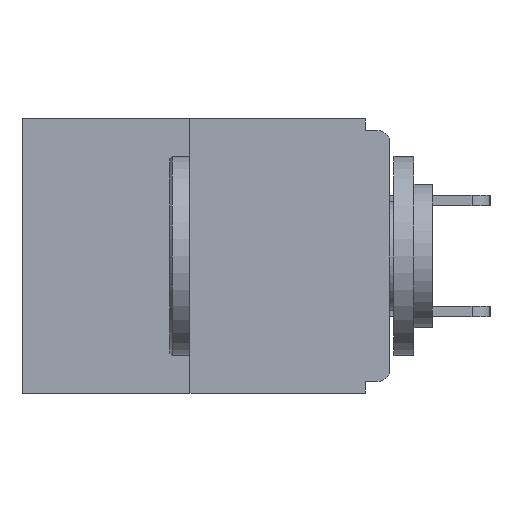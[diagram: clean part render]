
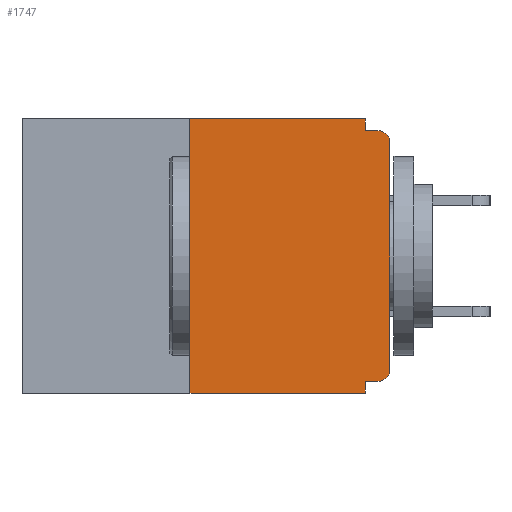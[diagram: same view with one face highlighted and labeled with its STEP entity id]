
A CAD part, left-side view. The second image highlights one B-rep face of the part: STEP entity #1747.
In plain terms, the highlighted planar face has unit normal (-1, 0, 0).
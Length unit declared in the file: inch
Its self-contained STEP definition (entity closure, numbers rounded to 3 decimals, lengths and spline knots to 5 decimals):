
#336 = CARTESIAN_POINT ( 'NONE',  ( 0., 0., 0. ) ) ;
#378 = EDGE_CURVE ( 'NONE', #7450, #7060, #9176, .T. ) ;
#493 = ORIENTED_EDGE ( 'NONE', *, *, #6042, .T. ) ;
#903 = CARTESIAN_POINT ( 'NONE',  ( 0., 0.015, -0.328 ) ) ;
#1571 = AXIS2_PLACEMENT_3D ( 'NONE', #9705, #12685, #5199 ) ;
#1747 = ADVANCED_FACE ( 'NONE', ( #12471 ), #16824, .F. ) ;
#1782 = ORIENTED_EDGE ( 'NONE', *, *, #12247, .F. ) ;
#1914 = VECTOR ( 'NONE', #4579, 39.37008 ) ;
#2179 = ORIENTED_EDGE ( 'NONE', *, *, #2939, .T. ) ;
#2742 = CARTESIAN_POINT ( 'NONE',  ( 0., 0.031, 0. ) ) ;
#2891 = VECTOR ( 'NONE', #10125, 39.37008 ) ;
#2907 = ORIENTED_EDGE ( 'NONE', *, *, #17609, .F. ) ;
#2908 = CIRCLE ( 'NONE', #16454, 0.015 ) ;
#2939 = EDGE_CURVE ( 'NONE', #8677, #5398, #2908, .T. ) ;
#3215 = DIRECTION ( 'NONE',  ( 0., -1., 0. ) ) ;
#3531 = LINE ( 'NONE', #6331, #19119 ) ;
#3634 = EDGE_LOOP ( 'NONE', ( #19291, #2907, #9939, #10907, #9017, #2179, #13256, #493, #1782, #12936 ) ) ;
#3779 = LINE ( 'NONE', #4654, #7376 ) ;
#3842 = VERTEX_POINT ( 'NONE', #15875 ) ;
#4537 = VERTEX_POINT ( 'NONE', #10192 ) ;
#4558 = VERTEX_POINT ( 'NONE', #11864 ) ;
#4579 = DIRECTION ( 'NONE',  ( 0., 1., 0. ) ) ;
#4654 = CARTESIAN_POINT ( 'NONE',  ( 0., 0.46, -0.343 ) ) ;
#5199 = DIRECTION ( 'NONE',  ( 0., 0., -1. ) ) ;
#5398 = VERTEX_POINT ( 'NONE', #12052 ) ;
#5694 = VERTEX_POINT ( 'NONE', #8526 ) ;
#5939 = LINE ( 'NONE', #18238, #1914 ) ;
#6042 = EDGE_CURVE ( 'NONE', #4558, #12372, #14712, .T. ) ;
#6188 = DIRECTION ( 'NONE',  ( 0., -1., 0. ) ) ;
#6326 = DIRECTION ( 'NONE',  ( -1., 0., 0. ) ) ;
#6331 = CARTESIAN_POINT ( 'NONE',  ( 0., 0., -0.015 ) ) ;
#6451 = LINE ( 'NONE', #18977, #2891 ) ;
#6812 = EDGE_CURVE ( 'NONE', #5398, #4558, #17959, .T. ) ;
#7060 = VERTEX_POINT ( 'NONE', #12876 ) ;
#7376 = VECTOR ( 'NONE', #6188, 39.37008 ) ;
#7450 = VERTEX_POINT ( 'NONE', #12485 ) ;
#7840 = VECTOR ( 'NONE', #17585, 39.37008 ) ;
#7907 = DIRECTION ( 'NONE',  ( 0., 0., -1. ) ) ;
#8076 = LINE ( 'NONE', #8389, #7840 ) ;
#8389 = CARTESIAN_POINT ( 'NONE',  ( 0., 0.25, 0. ) ) ;
#8526 = CARTESIAN_POINT ( 'NONE',  ( 0., 0.25, -0.343 ) ) ;
#8677 = VERTEX_POINT ( 'NONE', #903 ) ;
#8842 = LINE ( 'NONE', #2742, #9540 ) ;
#9017 = ORIENTED_EDGE ( 'NONE', *, *, #17894, .F. ) ;
#9176 = LINE ( 'NONE', #15212, #18813 ) ;
#9540 = VECTOR ( 'NONE', #15038, 39.37008 ) ;
#9705 = CARTESIAN_POINT ( 'NONE',  ( 0., 0.015, -0.03 ) ) ;
#9915 = CARTESIAN_POINT ( 'NONE',  ( 0., 0.031, -0.015 ) ) ;
#9939 = ORIENTED_EDGE ( 'NONE', *, *, #17833, .T. ) ;
#10125 = DIRECTION ( 'NONE',  ( 0., 0., -1. ) ) ;
#10192 = CARTESIAN_POINT ( 'NONE',  ( 0., 0.031, -0.343 ) ) ;
#10907 = ORIENTED_EDGE ( 'NONE', *, *, #16647, .F. ) ;
#11081 = EDGE_CURVE ( 'NONE', #7060, #14010, #8842, .T. ) ;
#11864 = CARTESIAN_POINT ( 'NONE',  ( 0., 0., -0.03 ) ) ;
#12052 = CARTESIAN_POINT ( 'NONE',  ( 0., 0., -0.313 ) ) ;
#12247 = EDGE_CURVE ( 'NONE', #14010, #12372, #3531, .T. ) ;
#12372 = VERTEX_POINT ( 'NONE', #18634 ) ;
#12471 = FACE_OUTER_BOUND ( 'NONE', #3634, .T. ) ;
#12485 = CARTESIAN_POINT ( 'NONE',  ( 0., 0.25, 0. ) ) ;
#12623 = DIRECTION ( 'NONE',  ( 0., 0., 1. ) ) ;
#12685 = DIRECTION ( 'NONE',  ( -1., 0., 0. ) ) ;
#12876 = CARTESIAN_POINT ( 'NONE',  ( 0., 0.031, 0. ) ) ;
#12936 = ORIENTED_EDGE ( 'NONE', *, *, #11081, .F. ) ;
#13256 = ORIENTED_EDGE ( 'NONE', *, *, #6812, .T. ) ;
#13505 = DIRECTION ( 'NONE',  ( 0., -1., 0. ) ) ;
#13897 = DIRECTION ( 'NONE',  ( 1., 0., 0. ) ) ;
#14010 = VERTEX_POINT ( 'NONE', #9915 ) ;
#14712 = CIRCLE ( 'NONE', #1571, 0.015 ) ;
#15038 = DIRECTION ( 'NONE',  ( 0., 0., -1. ) ) ;
#15212 = CARTESIAN_POINT ( 'NONE',  ( 0., 0.46, 0. ) ) ;
#15236 = CARTESIAN_POINT ( 'NONE',  ( 0., 0.015, -0.313 ) ) ;
#15384 = DIRECTION ( 'NONE',  ( 0., 0., -1. ) ) ;
#15875 = CARTESIAN_POINT ( 'NONE',  ( 0., 0.031, -0.328 ) ) ;
#15930 = AXIS2_PLACEMENT_3D ( 'NONE', #17081, #13897, #15384 ) ;
#16454 = AXIS2_PLACEMENT_3D ( 'NONE', #15236, #6326, #7907 ) ;
#16647 = EDGE_CURVE ( 'NONE', #3842, #4537, #6451, .T. ) ;
#16824 = PLANE ( 'NONE',  #15930 ) ;
#17081 = CARTESIAN_POINT ( 'NONE',  ( 0., 0.46, 0. ) ) ;
#17585 = DIRECTION ( 'NONE',  ( 0., 0., 1. ) ) ;
#17609 = EDGE_CURVE ( 'NONE', #5694, #7450, #8076, .T. ) ;
#17833 = EDGE_CURVE ( 'NONE', #5694, #4537, #3779, .T. ) ;
#17894 = EDGE_CURVE ( 'NONE', #8677, #3842, #5939, .T. ) ;
#17959 = LINE ( 'NONE', #336, #18898 ) ;
#18238 = CARTESIAN_POINT ( 'NONE',  ( 0., 0., -0.328 ) ) ;
#18634 = CARTESIAN_POINT ( 'NONE',  ( 0., 0.015, -0.015 ) ) ;
#18813 = VECTOR ( 'NONE', #13505, 39.37008 ) ;
#18898 = VECTOR ( 'NONE', #12623, 39.37008 ) ;
#18977 = CARTESIAN_POINT ( 'NONE',  ( 0., 0.031, -0.343 ) ) ;
#19119 = VECTOR ( 'NONE', #3215, 39.37008 ) ;
#19291 = ORIENTED_EDGE ( 'NONE', *, *, #378, .F. ) ;
